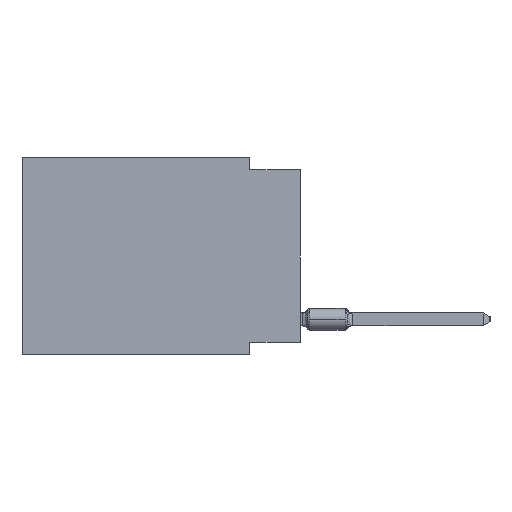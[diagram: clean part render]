
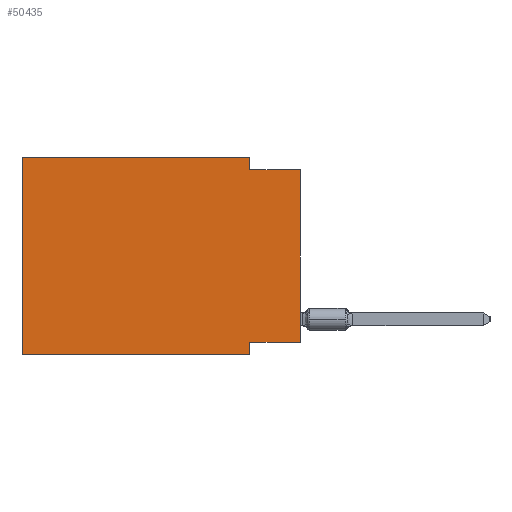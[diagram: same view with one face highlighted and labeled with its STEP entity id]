
A CAD part, left-side view. The second image highlights one B-rep face of the part: STEP entity #50435.
In plain terms, the highlighted planar face has unit normal (-1, 0, 0).
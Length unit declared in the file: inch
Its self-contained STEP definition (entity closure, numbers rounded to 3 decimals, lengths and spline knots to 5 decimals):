
#1775 = PLANE ( 'NONE',  #49247 ) ;
#2038 = DIRECTION ( 'NONE',  ( 0., 0., 1. ) ) ;
#2862 = LINE ( 'NONE', #32218, #55231 ) ;
#3195 = LINE ( 'NONE', #26151, #17465 ) ;
#3561 = VERTEX_POINT ( 'NONE', #38018 ) ;
#6116 = DIRECTION ( 'NONE',  ( 0., 0., -1. ) ) ;
#8541 = LINE ( 'NONE', #41658, #39962 ) ;
#8921 = CARTESIAN_POINT ( 'NONE',  ( 0., 0.55, 0. ) ) ;
#10352 = CARTESIAN_POINT ( 'NONE',  ( 0., 0.1, 0. ) ) ;
#14548 = DIRECTION ( 'NONE',  ( 0., 1., 0. ) ) ;
#14997 = VERTEX_POINT ( 'NONE', #68351 ) ;
#15477 = ORIENTED_EDGE ( 'NONE', *, *, #56031, .T. ) ;
#15482 = VECTOR ( 'NONE', #23096, 39.37008 ) ;
#15767 = LINE ( 'NONE', #55293, #59603 ) ;
#16260 = DIRECTION ( 'NONE',  ( 0., -1., 0. ) ) ;
#17465 = VECTOR ( 'NONE', #49116, 39.37008 ) ;
#18456 = VECTOR ( 'NONE', #16260, 39.37008 ) ;
#23096 = DIRECTION ( 'NONE',  ( 0., 0., -1. ) ) ;
#25367 = VERTEX_POINT ( 'NONE', #60139 ) ;
#26151 = CARTESIAN_POINT ( 'NONE',  ( 0., 0.55, 0. ) ) ;
#28033 = EDGE_CURVE ( 'NONE', #60501, #47797, #65636, .T. ) ;
#29657 = CARTESIAN_POINT ( 'NONE',  ( 0., 0., -0.025 ) ) ;
#29942 = VERTEX_POINT ( 'NONE', #48122 ) ;
#30638 = CARTESIAN_POINT ( 'NONE',  ( 0., 0., 0. ) ) ;
#30651 = EDGE_CURVE ( 'NONE', #14997, #29942, #15767, .T. ) ;
#31246 = DIRECTION ( 'NONE',  ( 0., -1., 0. ) ) ;
#32218 = CARTESIAN_POINT ( 'NONE',  ( 0., 0., -0.365 ) ) ;
#37065 = CARTESIAN_POINT ( 'NONE',  ( 0., 0.55, -0.39 ) ) ;
#37707 = VERTEX_POINT ( 'NONE', #37065 ) ;
#37725 = VECTOR ( 'NONE', #2038, 39.37008 ) ;
#38018 = CARTESIAN_POINT ( 'NONE',  ( 0., 0.1, -0.365 ) ) ;
#38487 = LINE ( 'NONE', #39594, #18456 ) ;
#39594 = CARTESIAN_POINT ( 'NONE',  ( 0., 0., -0.025 ) ) ;
#39962 = VECTOR ( 'NONE', #71008, 39.37008 ) ;
#40028 = ORIENTED_EDGE ( 'NONE', *, *, #45737, .F. ) ;
#41477 = LINE ( 'NONE', #64051, #70373 ) ;
#41658 = CARTESIAN_POINT ( 'NONE',  ( 0., 0.55, -0.39 ) ) ;
#45737 = EDGE_CURVE ( 'NONE', #3561, #25367, #41477, .T. ) ;
#47701 = FACE_OUTER_BOUND ( 'NONE', #59492, .T. ) ;
#47797 = VERTEX_POINT ( 'NONE', #29657 ) ;
#48122 = CARTESIAN_POINT ( 'NONE',  ( 0., 0.1, 0. ) ) ;
#49116 = DIRECTION ( 'NONE',  ( 0., 0., 1. ) ) ;
#49247 = AXIS2_PLACEMENT_3D ( 'NONE', #8921, #70659, #60115 ) ;
#50435 = ADVANCED_FACE ( 'NONE', ( #47701 ), #1775, .F. ) ;
#51341 = LINE ( 'NONE', #10352, #15482 ) ;
#51434 = ORIENTED_EDGE ( 'NONE', *, *, #28033, .T. ) ;
#54234 = ORIENTED_EDGE ( 'NONE', *, *, #71741, .F. ) ;
#54953 = ORIENTED_EDGE ( 'NONE', *, *, #30651, .F. ) ;
#55231 = VECTOR ( 'NONE', #14548, 39.37008 ) ;
#55293 = CARTESIAN_POINT ( 'NONE',  ( 0., 0.55, 0. ) ) ;
#56031 = EDGE_CURVE ( 'NONE', #37707, #25367, #8541, .T. ) ;
#56700 = CARTESIAN_POINT ( 'NONE',  ( 0., 0.1, -0.025 ) ) ;
#58678 = EDGE_CURVE ( 'NONE', #66538, #47797, #38487, .T. ) ;
#59492 = EDGE_LOOP ( 'NONE', ( #51434, #61956, #71472, #54953, #73356, #15477, #40028, #54234 ) ) ;
#59603 = VECTOR ( 'NONE', #31246, 39.37008 ) ;
#60115 = DIRECTION ( 'NONE',  ( 0., 0., -1. ) ) ;
#60139 = CARTESIAN_POINT ( 'NONE',  ( 0., 0.1, -0.39 ) ) ;
#60501 = VERTEX_POINT ( 'NONE', #68844 ) ;
#61956 = ORIENTED_EDGE ( 'NONE', *, *, #58678, .F. ) ;
#64051 = CARTESIAN_POINT ( 'NONE',  ( 0., 0.1, -0.39 ) ) ;
#65636 = LINE ( 'NONE', #30638, #37725 ) ;
#65684 = EDGE_CURVE ( 'NONE', #37707, #14997, #3195, .T. ) ;
#66538 = VERTEX_POINT ( 'NONE', #56700 ) ;
#68351 = CARTESIAN_POINT ( 'NONE',  ( 0., 0.55, 0. ) ) ;
#68844 = CARTESIAN_POINT ( 'NONE',  ( 0., 0., -0.365 ) ) ;
#70373 = VECTOR ( 'NONE', #6116, 39.37008 ) ;
#70615 = EDGE_CURVE ( 'NONE', #29942, #66538, #51341, .T. ) ;
#70659 = DIRECTION ( 'NONE',  ( 1., 0., 0. ) ) ;
#71008 = DIRECTION ( 'NONE',  ( 0., -1., 0. ) ) ;
#71472 = ORIENTED_EDGE ( 'NONE', *, *, #70615, .F. ) ;
#71741 = EDGE_CURVE ( 'NONE', #60501, #3561, #2862, .T. ) ;
#73356 = ORIENTED_EDGE ( 'NONE', *, *, #65684, .F. ) ;
